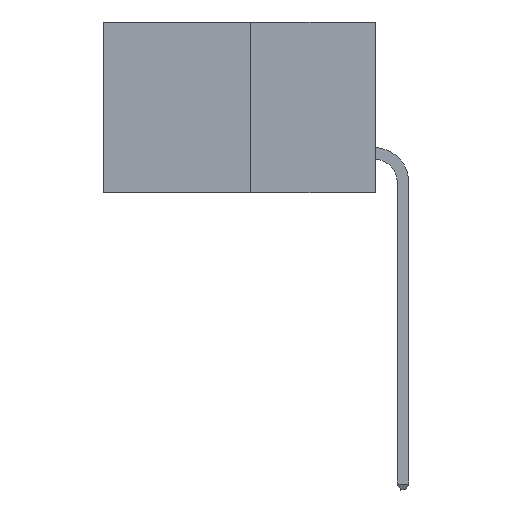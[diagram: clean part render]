
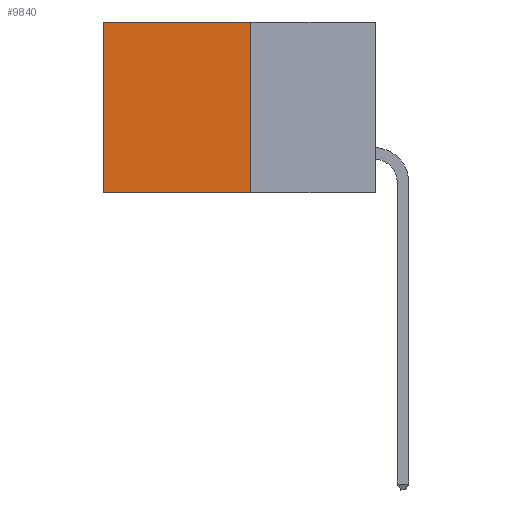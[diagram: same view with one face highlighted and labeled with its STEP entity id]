
A CAD part, left-side view. The second image highlights one B-rep face of the part: STEP entity #9840.
In plain terms, the highlighted planar face has unit normal (-1, 0, 0).
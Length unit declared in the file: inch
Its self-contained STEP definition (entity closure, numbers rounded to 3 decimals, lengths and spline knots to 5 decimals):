
#15 = VERTEX_POINT ( 'NONE', #6657 ) ;
#35 = DIRECTION ( 'NONE',  ( 0., 1., 0. ) ) ;
#378 = LINE ( 'NONE', #11749, #8295 ) ;
#1302 = CARTESIAN_POINT ( 'NONE',  ( 0.277, 0.27, -0.37 ) ) ;
#1561 = ORIENTED_EDGE ( 'NONE', *, *, #13090, .T. ) ;
#1671 = EDGE_CURVE ( 'NONE', #4753, #15, #378, .T. ) ;
#3453 = DIRECTION ( 'NONE',  ( 1., 0., 0. ) ) ;
#3536 = CARTESIAN_POINT ( 'NONE',  ( 0.277, 0.59, -0.37 ) ) ;
#3973 = CARTESIAN_POINT ( 'NONE',  ( 0.277, 0.27, 0. ) ) ;
#4256 = VECTOR ( 'NONE', #7818, 39.37008 ) ;
#4341 = CARTESIAN_POINT ( 'NONE',  ( 0.277, 0.27, -0.37 ) ) ;
#4753 = VERTEX_POINT ( 'NONE', #3973 ) ;
#5646 = CARTESIAN_POINT ( 'NONE',  ( 0.277, 0.27, 0. ) ) ;
#5770 = LINE ( 'NONE', #6383, #10752 ) ;
#6383 = CARTESIAN_POINT ( 'NONE',  ( 0.277, 0.59, -0.37 ) ) ;
#6638 = CARTESIAN_POINT ( 'NONE',  ( 0.277, 0.59, 0. ) ) ;
#6657 = CARTESIAN_POINT ( 'NONE',  ( 0.277, 0.27, -0.37 ) ) ;
#7278 = DIRECTION ( 'NONE',  ( 0., 0., -1. ) ) ;
#7596 = FACE_OUTER_BOUND ( 'NONE', #9997, .T. ) ;
#7818 = DIRECTION ( 'NONE',  ( 0., 1., 0. ) ) ;
#7915 = ORIENTED_EDGE ( 'NONE', *, *, #8181, .T. ) ;
#7963 = LINE ( 'NONE', #4341, #10427 ) ;
#8181 = EDGE_CURVE ( 'NONE', #4753, #9205, #12631, .T. ) ;
#8295 = VECTOR ( 'NONE', #7278, 39.37008 ) ;
#8840 = VERTEX_POINT ( 'NONE', #3536 ) ;
#9205 = VERTEX_POINT ( 'NONE', #6638 ) ;
#9633 = DIRECTION ( 'NONE',  ( 0., 0., -1. ) ) ;
#9840 = ADVANCED_FACE ( 'NONE', ( #7596 ), #12868, .F. ) ;
#9997 = EDGE_LOOP ( 'NONE', ( #1561, #10039, #12770, #7915 ) ) ;
#10039 = ORIENTED_EDGE ( 'NONE', *, *, #13135, .F. ) ;
#10427 = VECTOR ( 'NONE', #35, 39.37008 ) ;
#10752 = VECTOR ( 'NONE', #9633, 39.37008 ) ;
#10862 = DIRECTION ( 'NONE',  ( 0., 0., -1. ) ) ;
#11749 = CARTESIAN_POINT ( 'NONE',  ( 0.277, 0.27, -0.37 ) ) ;
#11829 = AXIS2_PLACEMENT_3D ( 'NONE', #1302, #3453, #10862 ) ;
#12631 = LINE ( 'NONE', #5646, #4256 ) ;
#12770 = ORIENTED_EDGE ( 'NONE', *, *, #1671, .F. ) ;
#12868 = PLANE ( 'NONE',  #11829 ) ;
#13090 = EDGE_CURVE ( 'NONE', #9205, #8840, #5770, .T. ) ;
#13135 = EDGE_CURVE ( 'NONE', #15, #8840, #7963, .T. ) ;
